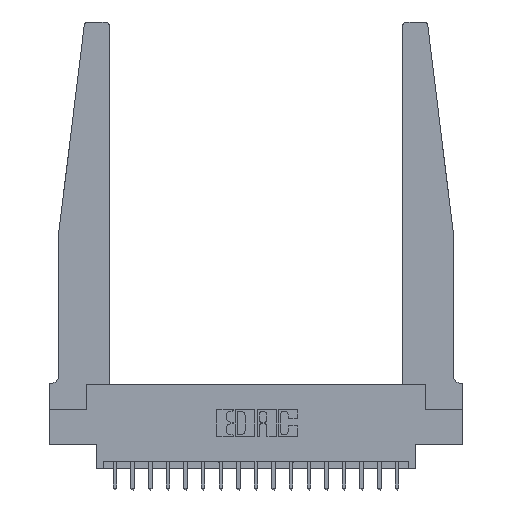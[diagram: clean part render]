
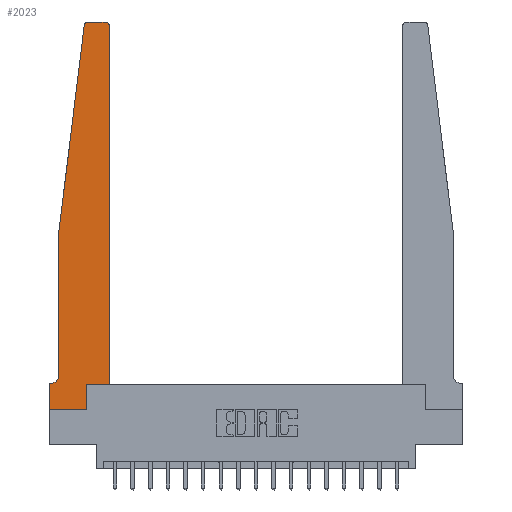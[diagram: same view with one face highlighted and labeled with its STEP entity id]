
A CAD part, top view. The second image highlights one B-rep face of the part: STEP entity #2023.
In plain terms, the highlighted planar face has unit normal (0, 0, 1).
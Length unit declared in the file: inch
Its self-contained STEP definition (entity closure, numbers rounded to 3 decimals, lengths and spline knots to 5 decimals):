
#158 = DIRECTION ( 'NONE',  ( 0., 0., 1. ) ) ;
#236 = EDGE_CURVE ( 'NONE', #7749, #8572, #10222, .T. ) ;
#427 = DIRECTION ( 'NONE',  ( 0., -1., 0. ) ) ;
#545 = EDGE_LOOP ( 'NONE', ( #12622, #3891, #18995, #18092, #4971, #18474, #5273, #11135, #14254, #9096, #15453, #2971 ) ) ;
#696 = EDGE_CURVE ( 'NONE', #12451, #10333, #8426, .T. ) ;
#814 = VECTOR ( 'NONE', #15221, 39.37008 ) ;
#915 = EDGE_CURVE ( 'NONE', #10333, #14820, #14480, .T. ) ;
#1362 = VECTOR ( 'NONE', #15021, 39.37008 ) ;
#1521 = DIRECTION ( 'NONE',  ( -0.122, -0.992, 0. ) ) ;
#1555 = VECTOR ( 'NONE', #4304, 39.37008 ) ;
#1740 = DIRECTION ( 'NONE',  ( 0., 0., 1. ) ) ;
#1841 = CARTESIAN_POINT ( 'NONE',  ( 0.24675, 2.72367, 0.37 ) ) ;
#1971 = CARTESIAN_POINT ( 'NONE',  ( 0., 0., 0.37 ) ) ;
#2023 = ADVANCED_FACE ( 'NONE', ( #4960 ), #18512, .T. ) ;
#2114 = LINE ( 'NONE', #9553, #19339 ) ;
#2345 = VECTOR ( 'NONE', #8258, 39.37008 ) ;
#2581 = LINE ( 'NONE', #16491, #1362 ) ;
#2971 = ORIENTED_EDGE ( 'NONE', *, *, #236, .T. ) ;
#3834 = VECTOR ( 'NONE', #10308, 39.37008 ) ;
#3891 = ORIENTED_EDGE ( 'NONE', *, *, #14529, .T. ) ;
#4236 = AXIS2_PLACEMENT_3D ( 'NONE', #18021, #15022, #18122 ) ;
#4304 = DIRECTION ( 'NONE',  ( 1., 0., 0. ) ) ;
#4930 = EDGE_CURVE ( 'NONE', #15863, #5566, #7119, .T. ) ;
#4960 = FACE_OUTER_BOUND ( 'NONE', #545, .T. ) ;
#4970 = CIRCLE ( 'NONE', #11718, 0.03 ) ;
#4971 = ORIENTED_EDGE ( 'NONE', *, *, #696, .T. ) ;
#5227 = VERTEX_POINT ( 'NONE', #6223 ) ;
#5273 = ORIENTED_EDGE ( 'NONE', *, *, #7522, .T. ) ;
#5386 = EDGE_CURVE ( 'NONE', #19002, #15863, #17712, .T. ) ;
#5496 = CARTESIAN_POINT ( 'NONE',  ( 0.2605, 0.18, 0.37 ) ) ;
#5566 = VERTEX_POINT ( 'NONE', #8090 ) ;
#5630 = CARTESIAN_POINT ( 'NONE',  ( 0.27653, 2.75, 0.37 ) ) ;
#5821 = CARTESIAN_POINT ( 'NONE',  ( 0.425, 0.18, 0.37 ) ) ;
#6009 = CARTESIAN_POINT ( 'NONE',  ( 0.25, 2.75, 0.37 ) ) ;
#6031 = VECTOR ( 'NONE', #1521, 39.37008 ) ;
#6223 = CARTESIAN_POINT ( 'NONE',  ( 0.065, 1.25, 0.37 ) ) ;
#6436 = LINE ( 'NONE', #12847, #17113 ) ;
#6836 = EDGE_CURVE ( 'NONE', #11061, #19002, #2581, .T. ) ;
#6870 = CARTESIAN_POINT ( 'NONE',  ( 0.065, 1.25, 0.37 ) ) ;
#6965 = CARTESIAN_POINT ( 'NONE',  ( 0.065, 0.1875, 0.37 ) ) ;
#7119 = LINE ( 'NONE', #5821, #1555 ) ;
#7281 = CARTESIAN_POINT ( 'NONE',  ( 0.015, 0.2375, 0.37 ) ) ;
#7522 = EDGE_CURVE ( 'NONE', #14820, #11061, #2114, .T. ) ;
#7749 = VERTEX_POINT ( 'NONE', #19468 ) ;
#8090 = CARTESIAN_POINT ( 'NONE',  ( 0.425, 0.18, 0.37 ) ) ;
#8258 = DIRECTION ( 'NONE',  ( -1., 0., 0. ) ) ;
#8426 = CIRCLE ( 'NONE', #11969, 0.05 ) ;
#8572 = VERTEX_POINT ( 'NONE', #9285 ) ;
#8737 = DIRECTION ( 'NONE',  ( 1., 0., 0. ) ) ;
#9096 = ORIENTED_EDGE ( 'NONE', *, *, #4930, .T. ) ;
#9285 = CARTESIAN_POINT ( 'NONE',  ( 0.395, 2.75, 0.37 ) ) ;
#9553 = CARTESIAN_POINT ( 'NONE',  ( 0., 0., 0.37 ) ) ;
#10222 = CIRCLE ( 'NONE', #4236, 0.03 ) ;
#10308 = DIRECTION ( 'NONE',  ( 0., 1., 0. ) ) ;
#10333 = VERTEX_POINT ( 'NONE', #17562 ) ;
#10365 = AXIS2_PLACEMENT_3D ( 'NONE', #11102, #158, #17184 ) ;
#10390 = DIRECTION ( 'NONE',  ( -1., 0., 0. ) ) ;
#10548 = CARTESIAN_POINT ( 'NONE',  ( 0.065, 1.25, 0.37 ) ) ;
#10757 = EDGE_CURVE ( 'NONE', #8572, #16483, #18024, .T. ) ;
#10879 = CARTESIAN_POINT ( 'NONE',  ( 0.27653, 2.72, 0.37 ) ) ;
#11061 = VERTEX_POINT ( 'NONE', #1971 ) ;
#11102 = CARTESIAN_POINT ( 'NONE',  ( 0., 0.1875, 0.37 ) ) ;
#11135 = ORIENTED_EDGE ( 'NONE', *, *, #6836, .T. ) ;
#11500 = LINE ( 'NONE', #6870, #17152 ) ;
#11718 = AXIS2_PLACEMENT_3D ( 'NONE', #10879, #1740, #8737 ) ;
#11879 = EDGE_CURVE ( 'NONE', #5566, #7749, #6436, .T. ) ;
#11969 = AXIS2_PLACEMENT_3D ( 'NONE', #7281, #19513, #10390 ) ;
#12451 = VERTEX_POINT ( 'NONE', #16379 ) ;
#12622 = ORIENTED_EDGE ( 'NONE', *, *, #10757, .T. ) ;
#12847 = CARTESIAN_POINT ( 'NONE',  ( 0.425, 0.18, 0.37 ) ) ;
#13928 = CARTESIAN_POINT ( 'NONE',  ( 0.2605, 0.18, 0.37 ) ) ;
#14141 = DIRECTION ( 'NONE',  ( 0., 1., 0. ) ) ;
#14254 = ORIENTED_EDGE ( 'NONE', *, *, #5386, .T. ) ;
#14464 = CARTESIAN_POINT ( 'NONE',  ( 0.2605, 0., 0.37 ) ) ;
#14480 = LINE ( 'NONE', #6965, #2345 ) ;
#14527 = VERTEX_POINT ( 'NONE', #1841 ) ;
#14529 = EDGE_CURVE ( 'NONE', #16483, #14527, #4970, .T. ) ;
#14820 = VERTEX_POINT ( 'NONE', #18185 ) ;
#15021 = DIRECTION ( 'NONE',  ( 1., 0., 0. ) ) ;
#15022 = DIRECTION ( 'NONE',  ( 0., 0., 1. ) ) ;
#15221 = DIRECTION ( 'NONE',  ( -1., 0., 0. ) ) ;
#15253 = LINE ( 'NONE', #10548, #6031 ) ;
#15453 = ORIENTED_EDGE ( 'NONE', *, *, #11879, .T. ) ;
#15863 = VERTEX_POINT ( 'NONE', #13928 ) ;
#16379 = CARTESIAN_POINT ( 'NONE',  ( 0.065, 0.2375, 0.37 ) ) ;
#16483 = VERTEX_POINT ( 'NONE', #5630 ) ;
#16491 = CARTESIAN_POINT ( 'NONE',  ( 0., 0., 0.37 ) ) ;
#17113 = VECTOR ( 'NONE', #14141, 39.37008 ) ;
#17152 = VECTOR ( 'NONE', #17587, 39.37008 ) ;
#17184 = DIRECTION ( 'NONE',  ( 1., 0., 0. ) ) ;
#17545 = EDGE_CURVE ( 'NONE', #5227, #12451, #11500, .T. ) ;
#17562 = CARTESIAN_POINT ( 'NONE',  ( 0.015, 0.1875, 0.37 ) ) ;
#17587 = DIRECTION ( 'NONE',  ( 0., -1., 0. ) ) ;
#17712 = LINE ( 'NONE', #5496, #3834 ) ;
#18021 = CARTESIAN_POINT ( 'NONE',  ( 0.395, 2.72, 0.37 ) ) ;
#18024 = LINE ( 'NONE', #6009, #814 ) ;
#18092 = ORIENTED_EDGE ( 'NONE', *, *, #17545, .T. ) ;
#18122 = DIRECTION ( 'NONE',  ( 1., 0., 0. ) ) ;
#18185 = CARTESIAN_POINT ( 'NONE',  ( 0., 0.1875, 0.37 ) ) ;
#18474 = ORIENTED_EDGE ( 'NONE', *, *, #915, .T. ) ;
#18512 = PLANE ( 'NONE',  #10365 ) ;
#18995 = ORIENTED_EDGE ( 'NONE', *, *, #19330, .T. ) ;
#19002 = VERTEX_POINT ( 'NONE', #14464 ) ;
#19330 = EDGE_CURVE ( 'NONE', #14527, #5227, #15253, .T. ) ;
#19339 = VECTOR ( 'NONE', #427, 39.37008 ) ;
#19468 = CARTESIAN_POINT ( 'NONE',  ( 0.425, 2.72, 0.37 ) ) ;
#19513 = DIRECTION ( 'NONE',  ( 0., 0., -1. ) ) ;
